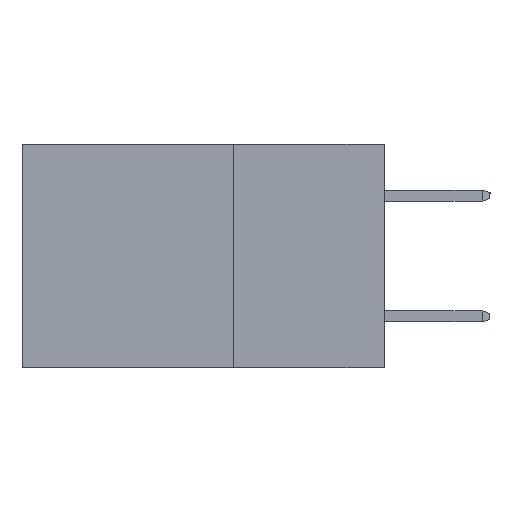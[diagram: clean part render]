
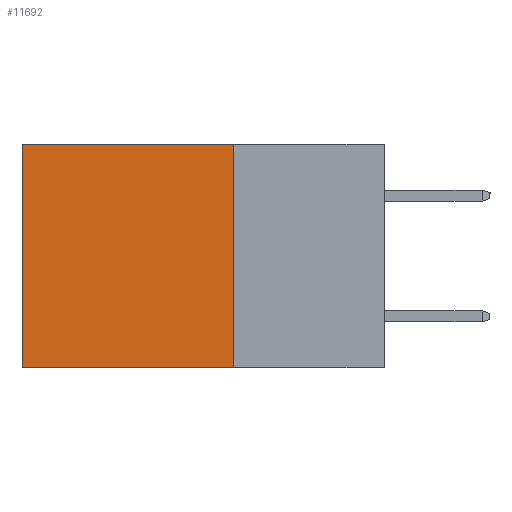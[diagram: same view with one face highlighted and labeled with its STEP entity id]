
A CAD part, left-side view. The second image highlights one B-rep face of the part: STEP entity #11692.
In plain terms, the highlighted planar face has unit normal (-1, 0, 0).
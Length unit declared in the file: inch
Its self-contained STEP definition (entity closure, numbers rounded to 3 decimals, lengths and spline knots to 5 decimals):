
#1 = EDGE_CURVE ( 'NONE', #5904, #10422, #4784, .T. ) ;
#161 = ORIENTED_EDGE ( 'NONE', *, *, #5099, .F. ) ;
#761 = CARTESIAN_POINT ( 'NONE',  ( 0.2615, 0.6, -0.37 ) ) ;
#855 = EDGE_LOOP ( 'NONE', ( #5353, #161, #10664, #6574 ) ) ;
#3026 = LINE ( 'NONE', #6837, #6589 ) ;
#3073 = LINE ( 'NONE', #6824, #6951 ) ;
#3395 = DIRECTION ( 'NONE',  ( 0., 1., 0. ) ) ;
#3485 = FACE_OUTER_BOUND ( 'NONE', #855, .T. ) ;
#3505 = VECTOR ( 'NONE', #5636, 39.37008 ) ;
#3587 = CARTESIAN_POINT ( 'NONE',  ( 0.2615, 0.25, 0. ) ) ;
#4258 = DIRECTION ( 'NONE',  ( 1., 0., 0. ) ) ;
#4742 = VERTEX_POINT ( 'NONE', #761 ) ;
#4784 = LINE ( 'NONE', #3587, #3505 ) ;
#5099 = EDGE_CURVE ( 'NONE', #9951, #4742, #6203, .T. ) ;
#5353 = ORIENTED_EDGE ( 'NONE', *, *, #11109, .T. ) ;
#5636 = DIRECTION ( 'NONE',  ( 0., 1., 0. ) ) ;
#5904 = VERTEX_POINT ( 'NONE', #9646 ) ;
#6117 = PLANE ( 'NONE',  #9175 ) ;
#6203 = LINE ( 'NONE', #9989, #8903 ) ;
#6301 = CARTESIAN_POINT ( 'NONE',  ( 0.2615, 0.6, 0. ) ) ;
#6574 = ORIENTED_EDGE ( 'NONE', *, *, #1, .T. ) ;
#6589 = VECTOR ( 'NONE', #10624, 39.37008 ) ;
#6824 = CARTESIAN_POINT ( 'NONE',  ( 0.2615, 0.25, -0.37 ) ) ;
#6837 = CARTESIAN_POINT ( 'NONE',  ( 0.2615, 0.6, -0.37 ) ) ;
#6951 = VECTOR ( 'NONE', #9682, 39.37008 ) ;
#8903 = VECTOR ( 'NONE', #3395, 39.37008 ) ;
#9175 = AXIS2_PLACEMENT_3D ( 'NONE', #11836, #4258, #10911 ) ;
#9515 = EDGE_CURVE ( 'NONE', #5904, #9951, #3073, .T. ) ;
#9646 = CARTESIAN_POINT ( 'NONE',  ( 0.2615, 0.25, 0. ) ) ;
#9682 = DIRECTION ( 'NONE',  ( 0., 0., -1. ) ) ;
#9951 = VERTEX_POINT ( 'NONE', #10349 ) ;
#9989 = CARTESIAN_POINT ( 'NONE',  ( 0.2615, 0.25, -0.37 ) ) ;
#10349 = CARTESIAN_POINT ( 'NONE',  ( 0.2615, 0.25, -0.37 ) ) ;
#10422 = VERTEX_POINT ( 'NONE', #6301 ) ;
#10624 = DIRECTION ( 'NONE',  ( 0., 0., -1. ) ) ;
#10664 = ORIENTED_EDGE ( 'NONE', *, *, #9515, .F. ) ;
#10911 = DIRECTION ( 'NONE',  ( 0., 0., -1. ) ) ;
#11109 = EDGE_CURVE ( 'NONE', #10422, #4742, #3026, .T. ) ;
#11692 = ADVANCED_FACE ( 'NONE', ( #3485 ), #6117, .F. ) ;
#11836 = CARTESIAN_POINT ( 'NONE',  ( 0.2615, 0.25, -0.37 ) ) ;
